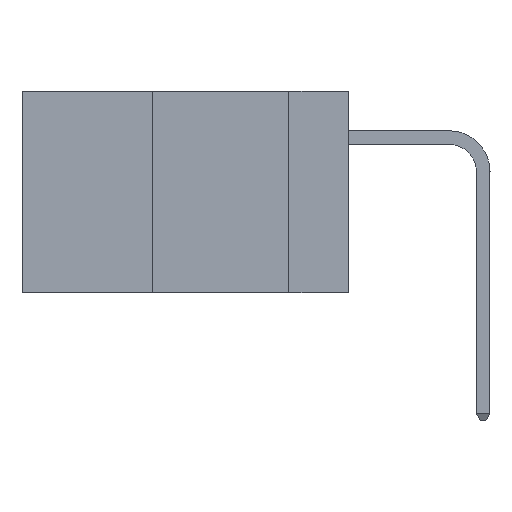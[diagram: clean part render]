
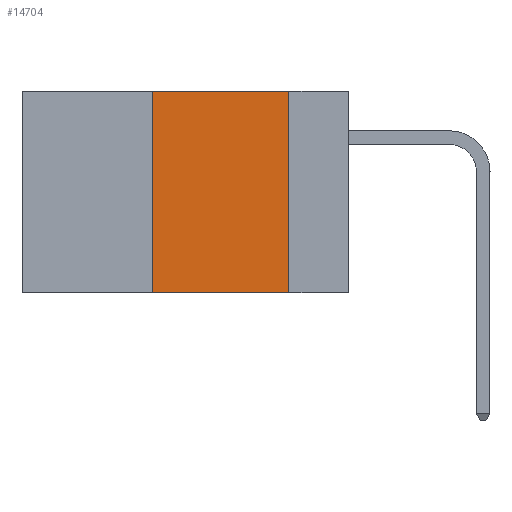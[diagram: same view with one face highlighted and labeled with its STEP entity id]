
A CAD part, left-side view. The second image highlights one B-rep face of the part: STEP entity #14704.
In plain terms, the highlighted planar face has unit normal (-1, 0, 0).
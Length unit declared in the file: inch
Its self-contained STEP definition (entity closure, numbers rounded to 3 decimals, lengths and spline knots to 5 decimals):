
#36 = LINE ( 'NONE', #3466, #13780 ) ;
#226 = FACE_OUTER_BOUND ( 'NONE', #14529, .T. ) ;
#2578 = DIRECTION ( 'NONE',  ( 0., 0., 1. ) ) ;
#2579 = EDGE_CURVE ( 'NONE', #3392, #7581, #36, .T. ) ;
#2814 = CARTESIAN_POINT ( 'NONE',  ( 0., 0.6, 0. ) ) ;
#3392 = VERTEX_POINT ( 'NONE', #16731 ) ;
#3435 = CARTESIAN_POINT ( 'NONE',  ( 0., 0.6, 0. ) ) ;
#3466 = CARTESIAN_POINT ( 'NONE',  ( 0., 0.6, -0.37 ) ) ;
#4421 = VECTOR ( 'NONE', #7207, 39.37008 ) ;
#5117 = VECTOR ( 'NONE', #2578, 39.37008 ) ;
#5329 = CARTESIAN_POINT ( 'NONE',  ( 0., 0.36, 0. ) ) ;
#5501 = CARTESIAN_POINT ( 'NONE',  ( 0., 0.11, 0. ) ) ;
#5885 = CARTESIAN_POINT ( 'NONE',  ( 0., 0.11, 0. ) ) ;
#6036 = PLANE ( 'NONE',  #17011 ) ;
#6058 = CARTESIAN_POINT ( 'NONE',  ( 0., 0.11, -0.37 ) ) ;
#6281 = EDGE_CURVE ( 'NONE', #12297, #12392, #15522, .T. ) ;
#6718 = ORIENTED_EDGE ( 'NONE', *, *, #9577, .F. ) ;
#6736 = DIRECTION ( 'NONE',  ( 0., -1., 0. ) ) ;
#7207 = DIRECTION ( 'NONE',  ( 0., 0., -1. ) ) ;
#7581 = VERTEX_POINT ( 'NONE', #6058 ) ;
#8678 = DIRECTION ( 'NONE',  ( 0., 0., -1. ) ) ;
#9577 = EDGE_CURVE ( 'NONE', #3392, #12297, #12072, .T. ) ;
#11230 = DIRECTION ( 'NONE',  ( 1., 0., 0. ) ) ;
#11769 = LINE ( 'NONE', #5885, #4421 ) ;
#12072 = LINE ( 'NONE', #15560, #5117 ) ;
#12297 = VERTEX_POINT ( 'NONE', #5329 ) ;
#12392 = VERTEX_POINT ( 'NONE', #5501 ) ;
#13055 = EDGE_CURVE ( 'NONE', #12392, #7581, #11769, .T. ) ;
#13780 = VECTOR ( 'NONE', #16527, 39.37008 ) ;
#14206 = ORIENTED_EDGE ( 'NONE', *, *, #6281, .F. ) ;
#14529 = EDGE_LOOP ( 'NONE', ( #15745, #14206, #6718, #16245 ) ) ;
#14704 = ADVANCED_FACE ( 'NONE', ( #226 ), #6036, .F. ) ;
#15097 = VECTOR ( 'NONE', #6736, 39.37008 ) ;
#15522 = LINE ( 'NONE', #2814, #15097 ) ;
#15560 = CARTESIAN_POINT ( 'NONE',  ( 0., 0.36, 0. ) ) ;
#15745 = ORIENTED_EDGE ( 'NONE', *, *, #13055, .F. ) ;
#16245 = ORIENTED_EDGE ( 'NONE', *, *, #2579, .T. ) ;
#16527 = DIRECTION ( 'NONE',  ( 0., -1., 0. ) ) ;
#16731 = CARTESIAN_POINT ( 'NONE',  ( 0., 0.36, -0.37 ) ) ;
#17011 = AXIS2_PLACEMENT_3D ( 'NONE', #3435, #11230, #8678 ) ;
